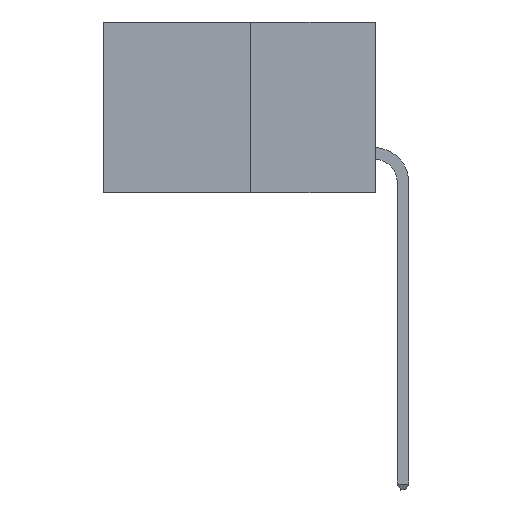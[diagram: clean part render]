
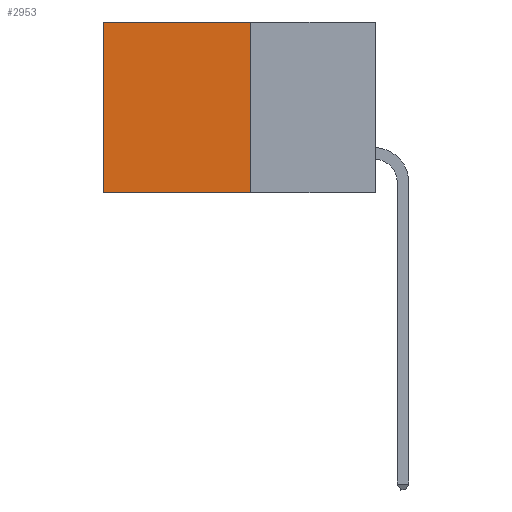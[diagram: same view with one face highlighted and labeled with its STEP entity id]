
A CAD part, left-side view. The second image highlights one B-rep face of the part: STEP entity #2953.
In plain terms, the highlighted planar face has unit normal (-1, 0, 0).
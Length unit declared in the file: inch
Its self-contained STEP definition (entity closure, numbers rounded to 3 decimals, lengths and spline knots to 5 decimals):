
#512 = ORIENTED_EDGE ( 'NONE', *, *, #8462, .T. ) ;
#579 = CARTESIAN_POINT ( 'NONE',  ( 0.277, 0.27, -0.37 ) ) ;
#857 = ORIENTED_EDGE ( 'NONE', *, *, #1397, .T. ) ;
#1397 = EDGE_CURVE ( 'NONE', #11399, #7154, #12940, .T. ) ;
#1734 = CARTESIAN_POINT ( 'NONE',  ( 0.277, 0.27, 0. ) ) ;
#2180 = FACE_OUTER_BOUND ( 'NONE', #4563, .T. ) ;
#2402 = LINE ( 'NONE', #4946, #11194 ) ;
#2806 = CARTESIAN_POINT ( 'NONE',  ( 0.277, 0.59, -0.37 ) ) ;
#2953 = ADVANCED_FACE ( 'NONE', ( #2180 ), #9080, .F. ) ;
#3278 = CARTESIAN_POINT ( 'NONE',  ( 0.277, 0.27, -0.37 ) ) ;
#4098 = VECTOR ( 'NONE', #8624, 39.37008 ) ;
#4448 = VECTOR ( 'NONE', #7496, 39.37008 ) ;
#4563 = EDGE_LOOP ( 'NONE', ( #512, #6680, #9677, #857 ) ) ;
#4946 = CARTESIAN_POINT ( 'NONE',  ( 0.277, 0.27, -0.37 ) ) ;
#5388 = CARTESIAN_POINT ( 'NONE',  ( 0.277, 0.27, -0.37 ) ) ;
#5715 = LINE ( 'NONE', #8549, #10983 ) ;
#6680 = ORIENTED_EDGE ( 'NONE', *, *, #7361, .F. ) ;
#7154 = VERTEX_POINT ( 'NONE', #12197 ) ;
#7361 = EDGE_CURVE ( 'NONE', #11677, #9363, #2402, .T. ) ;
#7496 = DIRECTION ( 'NONE',  ( 0., 0., -1. ) ) ;
#8462 = EDGE_CURVE ( 'NONE', #7154, #9363, #5715, .T. ) ;
#8549 = CARTESIAN_POINT ( 'NONE',  ( 0.277, 0.59, -0.37 ) ) ;
#8603 = AXIS2_PLACEMENT_3D ( 'NONE', #5388, #10959, #13901 ) ;
#8624 = DIRECTION ( 'NONE',  ( 0., 1., 0. ) ) ;
#8830 = CARTESIAN_POINT ( 'NONE',  ( 0.277, 0.27, 0. ) ) ;
#9080 = PLANE ( 'NONE',  #8603 ) ;
#9363 = VERTEX_POINT ( 'NONE', #2806 ) ;
#9677 = ORIENTED_EDGE ( 'NONE', *, *, #10780, .F. ) ;
#9790 = LINE ( 'NONE', #579, #4448 ) ;
#10780 = EDGE_CURVE ( 'NONE', #11399, #11677, #9790, .T. ) ;
#10959 = DIRECTION ( 'NONE',  ( 1., 0., 0. ) ) ;
#10983 = VECTOR ( 'NONE', #13369, 39.37008 ) ;
#11194 = VECTOR ( 'NONE', #13590, 39.37008 ) ;
#11399 = VERTEX_POINT ( 'NONE', #1734 ) ;
#11677 = VERTEX_POINT ( 'NONE', #3278 ) ;
#12197 = CARTESIAN_POINT ( 'NONE',  ( 0.277, 0.59, 0. ) ) ;
#12940 = LINE ( 'NONE', #8830, #4098 ) ;
#13369 = DIRECTION ( 'NONE',  ( 0., 0., -1. ) ) ;
#13590 = DIRECTION ( 'NONE',  ( 0., 1., 0. ) ) ;
#13901 = DIRECTION ( 'NONE',  ( 0., 0., -1. ) ) ;
